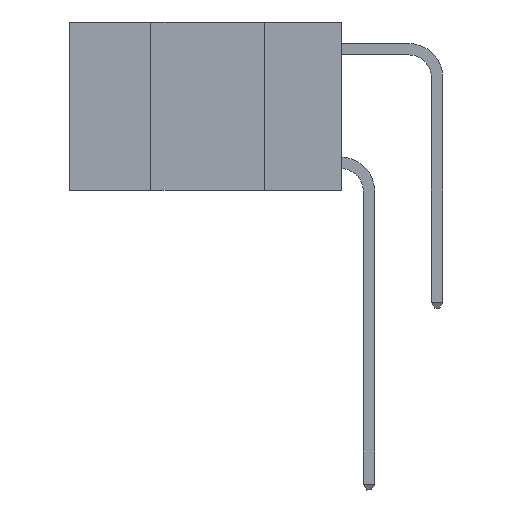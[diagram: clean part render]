
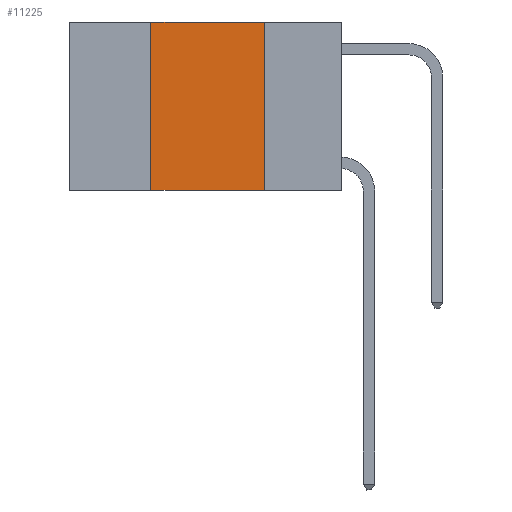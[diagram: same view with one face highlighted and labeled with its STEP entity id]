
A CAD part, left-side view. The second image highlights one B-rep face of the part: STEP entity #11225.
In plain terms, the highlighted planar face has unit normal (-1, 0, 0).
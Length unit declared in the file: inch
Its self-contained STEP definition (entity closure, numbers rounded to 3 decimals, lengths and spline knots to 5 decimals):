
#122 = ORIENTED_EDGE ( 'NONE', *, *, #15366, .F. ) ;
#807 = FACE_OUTER_BOUND ( 'NONE', #12753, .T. ) ;
#1346 = VERTEX_POINT ( 'NONE', #13284 ) ;
#2569 = LINE ( 'NONE', #17045, #8117 ) ;
#3405 = CARTESIAN_POINT ( 'NONE',  ( 0., 0.42, 0. ) ) ;
#4106 = VERTEX_POINT ( 'NONE', #13336 ) ;
#4959 = AXIS2_PLACEMENT_3D ( 'NONE', #17607, #17762, #10831 ) ;
#5825 = LINE ( 'NONE', #17226, #18299 ) ;
#6540 = DIRECTION ( 'NONE',  ( 0., -1., 0. ) ) ;
#6706 = EDGE_CURVE ( 'NONE', #12531, #14210, #2569, .T. ) ;
#6976 = ORIENTED_EDGE ( 'NONE', *, *, #6706, .F. ) ;
#8117 = VECTOR ( 'NONE', #15722, 39.37008 ) ;
#9532 = CARTESIAN_POINT ( 'NONE',  ( 0., 0.17, 0. ) ) ;
#10110 = DIRECTION ( 'NONE',  ( 0., -1., 0. ) ) ;
#10405 = VECTOR ( 'NONE', #6540, 39.37008 ) ;
#10831 = DIRECTION ( 'NONE',  ( 0., 0., -1. ) ) ;
#11225 = ADVANCED_FACE ( 'NONE', ( #807 ), #16391, .F. ) ;
#11771 = CARTESIAN_POINT ( 'NONE',  ( 0., 0.42, -0.37 ) ) ;
#11856 = LINE ( 'NONE', #13669, #10405 ) ;
#12531 = VERTEX_POINT ( 'NONE', #11771 ) ;
#12753 = EDGE_LOOP ( 'NONE', ( #16494, #122, #6976, #16254 ) ) ;
#13284 = CARTESIAN_POINT ( 'NONE',  ( 0., 0.17, -0.37 ) ) ;
#13336 = CARTESIAN_POINT ( 'NONE',  ( 0., 0.17, 0. ) ) ;
#13422 = EDGE_CURVE ( 'NONE', #12531, #1346, #11856, .T. ) ;
#13669 = CARTESIAN_POINT ( 'NONE',  ( 0., 0.6, -0.37 ) ) ;
#14210 = VERTEX_POINT ( 'NONE', #3405 ) ;
#15366 = EDGE_CURVE ( 'NONE', #14210, #4106, #5825, .T. ) ;
#15722 = DIRECTION ( 'NONE',  ( 0., 0., 1. ) ) ;
#16254 = ORIENTED_EDGE ( 'NONE', *, *, #13422, .T. ) ;
#16391 = PLANE ( 'NONE',  #4959 ) ;
#16494 = ORIENTED_EDGE ( 'NONE', *, *, #18077, .F. ) ;
#17045 = CARTESIAN_POINT ( 'NONE',  ( 0., 0.42, 0. ) ) ;
#17226 = CARTESIAN_POINT ( 'NONE',  ( 0., 0.6, 0. ) ) ;
#17505 = DIRECTION ( 'NONE',  ( 0., 0., -1. ) ) ;
#17607 = CARTESIAN_POINT ( 'NONE',  ( 0., 0.6, 0. ) ) ;
#17650 = VECTOR ( 'NONE', #17505, 39.37008 ) ;
#17762 = DIRECTION ( 'NONE',  ( 1., 0., 0. ) ) ;
#17989 = LINE ( 'NONE', #9532, #17650 ) ;
#18077 = EDGE_CURVE ( 'NONE', #4106, #1346, #17989, .T. ) ;
#18299 = VECTOR ( 'NONE', #10110, 39.37008 ) ;
